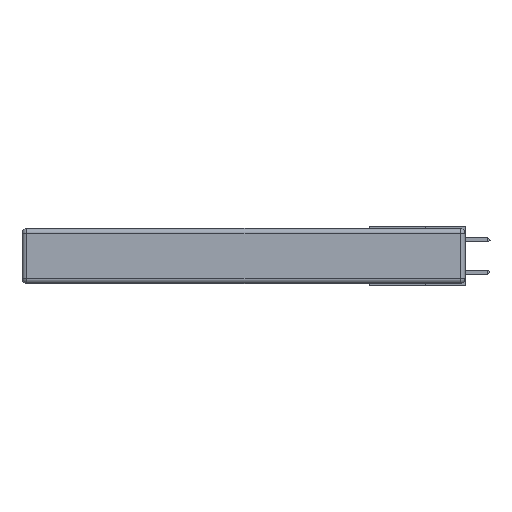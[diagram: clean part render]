
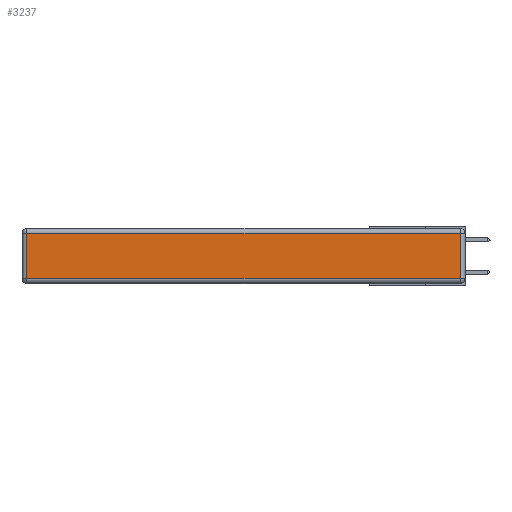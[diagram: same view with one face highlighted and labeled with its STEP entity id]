
A CAD part, left-side view. The second image highlights one B-rep face of the part: STEP entity #3237.
In plain terms, the highlighted planar face has unit normal (-1, 0, 0).
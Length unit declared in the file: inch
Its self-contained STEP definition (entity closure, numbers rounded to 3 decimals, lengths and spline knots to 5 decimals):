
#35 = EDGE_CURVE ( 'NONE', #1236, #15019, #5327, .T. ) ;
#211 = DIRECTION ( 'NONE',  ( -1., 0., 0. ) ) ;
#1236 = VERTEX_POINT ( 'NONE', #7690 ) ;
#2395 = CARTESIAN_POINT ( 'NONE',  ( 0., 0.03, -0.03 ) ) ;
#2723 = DIRECTION ( 'NONE',  ( 0., 0., 1. ) ) ;
#3134 = CARTESIAN_POINT ( 'NONE',  ( 0., 0., -0.313 ) ) ;
#3237 = ADVANCED_FACE ( 'NONE', ( #10057 ), #12380, .T. ) ;
#3537 = ORIENTED_EDGE ( 'NONE', *, *, #8511, .T. ) ;
#4096 = CARTESIAN_POINT ( 'NONE',  ( 0., 0.03, -0.343 ) ) ;
#4337 = VERTEX_POINT ( 'NONE', #2395 ) ;
#4673 = EDGE_LOOP ( 'NONE', ( #3537, #11241, #6169, #7147 ) ) ;
#5327 = LINE ( 'NONE', #15123, #8204 ) ;
#5614 = DIRECTION ( 'NONE',  ( 0., -1., 0. ) ) ;
#6169 = ORIENTED_EDGE ( 'NONE', *, *, #11018, .T. ) ;
#6176 = AXIS2_PLACEMENT_3D ( 'NONE', #14889, #211, #2723 ) ;
#7103 = CARTESIAN_POINT ( 'NONE',  ( 0., 2.75, -0.03 ) ) ;
#7147 = ORIENTED_EDGE ( 'NONE', *, *, #35, .T. ) ;
#7254 = VECTOR ( 'NONE', #12881, 39.37008 ) ;
#7382 = DIRECTION ( 'NONE',  ( 0., 1., 0. ) ) ;
#7690 = CARTESIAN_POINT ( 'NONE',  ( 0., 2.72, -0.03 ) ) ;
#7694 = CARTESIAN_POINT ( 'NONE',  ( 0., 0.03, -0.313 ) ) ;
#8204 = VECTOR ( 'NONE', #8910, 39.37008 ) ;
#8511 = EDGE_CURVE ( 'NONE', #15019, #9636, #14741, .T. ) ;
#8910 = DIRECTION ( 'NONE',  ( 0., 0., -1. ) ) ;
#9084 = VECTOR ( 'NONE', #7382, 39.37008 ) ;
#9459 = LINE ( 'NONE', #7103, #9084 ) ;
#9636 = VERTEX_POINT ( 'NONE', #7694 ) ;
#9964 = LINE ( 'NONE', #4096, #7254 ) ;
#10057 = FACE_OUTER_BOUND ( 'NONE', #4673, .T. ) ;
#11018 = EDGE_CURVE ( 'NONE', #4337, #1236, #9459, .T. ) ;
#11077 = VECTOR ( 'NONE', #5614, 39.37008 ) ;
#11241 = ORIENTED_EDGE ( 'NONE', *, *, #12389, .T. ) ;
#12380 = PLANE ( 'NONE',  #6176 ) ;
#12389 = EDGE_CURVE ( 'NONE', #9636, #4337, #9964, .T. ) ;
#12634 = CARTESIAN_POINT ( 'NONE',  ( 0., 2.72, -0.313 ) ) ;
#12881 = DIRECTION ( 'NONE',  ( 0., 0., 1. ) ) ;
#14741 = LINE ( 'NONE', #3134, #11077 ) ;
#14889 = CARTESIAN_POINT ( 'NONE',  ( 0., 0., -0.343 ) ) ;
#15019 = VERTEX_POINT ( 'NONE', #12634 ) ;
#15123 = CARTESIAN_POINT ( 'NONE',  ( 0., 2.72, -0.343 ) ) ;
